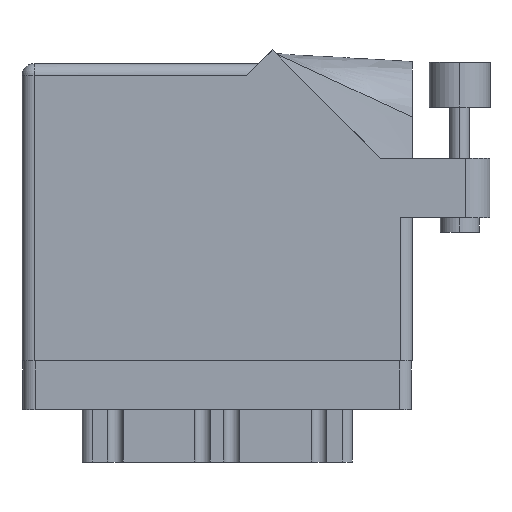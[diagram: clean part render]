
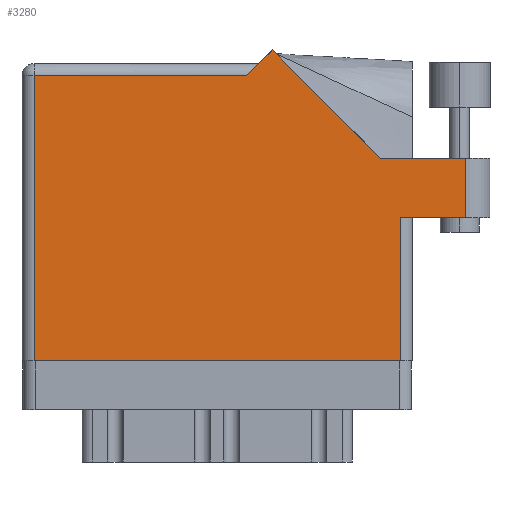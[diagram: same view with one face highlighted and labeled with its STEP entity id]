
A CAD part, front view. The second image highlights one B-rep face of the part: STEP entity #3280.
In plain terms, the highlighted face is planar.
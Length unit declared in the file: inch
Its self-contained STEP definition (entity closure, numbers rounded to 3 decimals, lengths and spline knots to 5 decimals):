
#620 = CARTESIAN_POINT ( 'NONE',  ( 1.948, 0.737, 0. ) ) ;
#1007 = LINE ( 'NONE', #620, #27477 ) ;
#1030 = CARTESIAN_POINT ( 'NONE',  ( 1.84442, 1.044, 0. ) ) ;
#1313 = AXIS2_PLACEMENT_3D ( 'NONE', #33519, #18951, #37044 ) ;
#1627 = CARTESIAN_POINT ( 'NONE',  ( 0.062, 0., 0. ) ) ;
#2282 = VECTOR ( 'NONE', #37017, 39.37008 ) ;
#2346 = VERTEX_POINT ( 'NONE', #35099 ) ;
#2414 = EDGE_CURVE ( 'NONE', #36929, #2346, #11291, .T. ) ;
#2798 = ORIENTED_EDGE ( 'NONE', *, *, #22841, .T. ) ;
#3280 = ADVANCED_FACE ( 'NONE', ( #25066 ), #22108, .F. ) ;
#4206 = EDGE_CURVE ( 'NONE', #27757, #28632, #1007, .T. ) ;
#5253 = EDGE_CURVE ( 'NONE', #28632, #36929, #37871, .T. ) ;
#5695 = EDGE_CURVE ( 'NONE', #33991, #27757, #20270, .T. ) ;
#5985 = CARTESIAN_POINT ( 'NONE',  ( 0.062, 0., 0. ) ) ;
#6571 = CARTESIAN_POINT ( 'NONE',  ( 0., 1.468, 0. ) ) ;
#7013 = ORIENTED_EDGE ( 'NONE', *, *, #2414, .T. ) ;
#7863 = CARTESIAN_POINT ( 'NONE',  ( 0.062, 1.468, 0. ) ) ;
#7898 = CARTESIAN_POINT ( 'NONE',  ( 1.217, 1.53, 0. ) ) ;
#9817 = ORIENTED_EDGE ( 'NONE', *, *, #17409, .T. ) ;
#10409 = ORIENTED_EDGE ( 'NONE', *, *, #5695, .T. ) ;
#10885 = CARTESIAN_POINT ( 'NONE',  ( 1.84442, 1.044, 0. ) ) ;
#10901 = CARTESIAN_POINT ( 'NONE',  ( 2.285, 1.044, 0. ) ) ;
#11026 = CARTESIAN_POINT ( 'NONE',  ( 1.28771, 1.60071, 0. ) ) ;
#11291 = LINE ( 'NONE', #10901, #38295 ) ;
#11398 = DIRECTION ( 'NONE',  ( 1., 0., 0. ) ) ;
#12972 = DIRECTION ( 'NONE',  ( 0., 1., 0. ) ) ;
#13497 = DIRECTION ( 'NONE',  ( -1., 0., 0. ) ) ;
#14477 = VECTOR ( 'NONE', #11398, 39.37008 ) ;
#15499 = VERTEX_POINT ( 'NONE', #1030 ) ;
#15849 = VECTOR ( 'NONE', #31149, 39.37008 ) ;
#16001 = LINE ( 'NONE', #6571, #15849 ) ;
#16099 = VECTOR ( 'NONE', #17873, 39.37008 ) ;
#16427 = EDGE_CURVE ( 'NONE', #2346, #15499, #37303, .T. ) ;
#16790 = LINE ( 'NONE', #10885, #24489 ) ;
#16997 = CARTESIAN_POINT ( 'NONE',  ( 1.948, 0.737, 0. ) ) ;
#17248 = ORIENTED_EDGE ( 'NONE', *, *, #16427, .T. ) ;
#17409 = EDGE_CURVE ( 'NONE', #19181, #33991, #33877, .T. ) ;
#17506 = EDGE_CURVE ( 'NONE', #23175, #26364, #17677, .T. ) ;
#17677 = LINE ( 'NONE', #7898, #16099 ) ;
#17873 = DIRECTION ( 'NONE',  ( -0.707, -0.707, 0. ) ) ;
#18951 = DIRECTION ( 'NONE',  ( 0., 0., -1. ) ) ;
#19181 = VERTEX_POINT ( 'NONE', #7863 ) ;
#19792 = CARTESIAN_POINT ( 'NONE',  ( 2.285, 0.737, 0. ) ) ;
#19878 = CARTESIAN_POINT ( 'NONE',  ( 0., 0., 0. ) ) ;
#20270 = LINE ( 'NONE', #19878, #14477 ) ;
#20783 = CARTESIAN_POINT ( 'NONE',  ( 1.155, 1.468, 0. ) ) ;
#22108 = PLANE ( 'NONE',  #1313 ) ;
#22841 = EDGE_CURVE ( 'NONE', #15499, #23175, #16790, .T. ) ;
#23062 = ORIENTED_EDGE ( 'NONE', *, *, #4206, .T. ) ;
#23175 = VERTEX_POINT ( 'NONE', #11026 ) ;
#23391 = CARTESIAN_POINT ( 'NONE',  ( 1.948, 0., 0. ) ) ;
#24489 = VECTOR ( 'NONE', #25659, 39.37008 ) ;
#25066 = FACE_OUTER_BOUND ( 'NONE', #28495, .T. ) ;
#25269 = VECTOR ( 'NONE', #25494, 39.37008 ) ;
#25494 = DIRECTION ( 'NONE',  ( 1., 0., 0. ) ) ;
#25659 = DIRECTION ( 'NONE',  ( -0.707, 0.707, 0. ) ) ;
#26364 = VERTEX_POINT ( 'NONE', #20783 ) ;
#27197 = EDGE_CURVE ( 'NONE', #26364, #19181, #16001, .T. ) ;
#27477 = VECTOR ( 'NONE', #12972, 39.37008 ) ;
#27757 = VERTEX_POINT ( 'NONE', #23391 ) ;
#27762 = ORIENTED_EDGE ( 'NONE', *, *, #17506, .T. ) ;
#28495 = EDGE_LOOP ( 'NONE', ( #30451, #7013, #17248, #2798, #27762, #35573, #9817, #10409, #23062 ) ) ;
#28632 = VERTEX_POINT ( 'NONE', #16997 ) ;
#30451 = ORIENTED_EDGE ( 'NONE', *, *, #5253, .T. ) ;
#31149 = DIRECTION ( 'NONE',  ( -1., 0., 0. ) ) ;
#31179 = CARTESIAN_POINT ( 'NONE',  ( 2.01, 0.737, 0. ) ) ;
#33519 = CARTESIAN_POINT ( 'NONE',  ( 0., 1.53, 0. ) ) ;
#33877 = LINE ( 'NONE', #1627, #2282 ) ;
#33991 = VERTEX_POINT ( 'NONE', #5985 ) ;
#35099 = CARTESIAN_POINT ( 'NONE',  ( 2.285, 1.044, 0. ) ) ;
#35573 = ORIENTED_EDGE ( 'NONE', *, *, #27197, .T. ) ;
#36929 = VERTEX_POINT ( 'NONE', #19792 ) ;
#37017 = DIRECTION ( 'NONE',  ( 0., -1., 0. ) ) ;
#37044 = DIRECTION ( 'NONE',  ( -1., 0., 0. ) ) ;
#37303 = LINE ( 'NONE', #37898, #38026 ) ;
#37871 = LINE ( 'NONE', #31179, #25269 ) ;
#37898 = CARTESIAN_POINT ( 'NONE',  ( 2.41, 1.044, 0. ) ) ;
#38026 = VECTOR ( 'NONE', #13497, 39.37008 ) ;
#38242 = DIRECTION ( 'NONE',  ( 0., 1., 0. ) ) ;
#38295 = VECTOR ( 'NONE', #38242, 39.37008 ) ;
